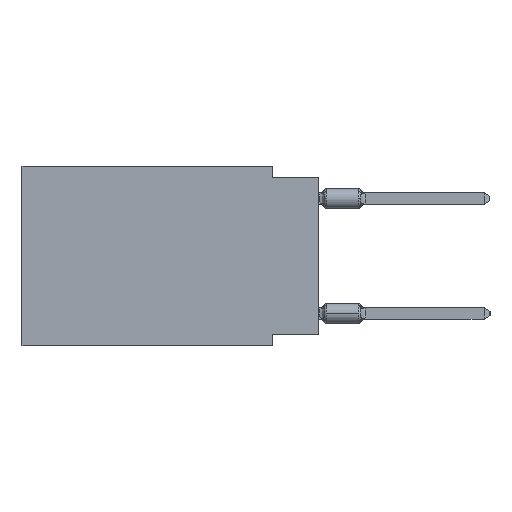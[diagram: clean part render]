
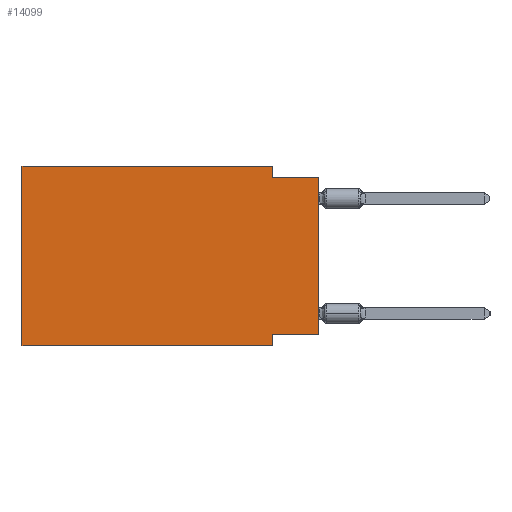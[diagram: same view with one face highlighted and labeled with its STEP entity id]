
A CAD part, left-side view. The second image highlights one B-rep face of the part: STEP entity #14099.
In plain terms, the highlighted planar face has unit normal (-1, 0, 0).
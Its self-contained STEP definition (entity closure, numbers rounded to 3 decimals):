
#2084 = ORIENTED_EDGE ( 'NONE', *, *, #8883, .F. ) ;
#2265 = VERTEX_POINT ( 'NONE', #6997 ) ;
#2411 = LINE ( 'NONE', #27732, #25319 ) ;
#3256 = DIRECTION ( 'NONE',  ( 0., -1., 0. ) ) ;
#3258 = ORIENTED_EDGE ( 'NONE', *, *, #47638, .T. ) ;
#3828 = VECTOR ( 'NONE', #37073, 1000. ) ;
#6430 = CARTESIAN_POINT ( 'NONE',  ( 0., 0., 0. ) ) ;
#6997 = CARTESIAN_POINT ( 'NONE',  ( 0., 2.54, -9.271 ) ) ;
#7080 = LINE ( 'NONE', #24614, #47276 ) ;
#8883 = EDGE_CURVE ( 'NONE', #46232, #43087, #38682, .T. ) ;
#8958 = EDGE_LOOP ( 'NONE', ( #43177, #30662, #22800, #29225, #2084, #3258, #28585, #29374 ) ) ;
#9475 = EDGE_CURVE ( 'NONE', #43087, #46721, #20190, .T. ) ;
#9549 = VECTOR ( 'NONE', #43375, 1000. ) ;
#9982 = LINE ( 'NONE', #18326, #9549 ) ;
#10958 = CARTESIAN_POINT ( 'NONE',  ( 0., 0., -9.271 ) ) ;
#11141 = EDGE_CURVE ( 'NONE', #47930, #27994, #48956, .T. ) ;
#13246 = VECTOR ( 'NONE', #52316, 1000. ) ;
#14099 = ADVANCED_FACE ( 'NONE', ( #23675 ), #27549, .F. ) ;
#14908 = CARTESIAN_POINT ( 'NONE',  ( 0., 16.383, 0. ) ) ;
#15680 = CARTESIAN_POINT ( 'NONE',  ( 0., 0., -9.271 ) ) ;
#15889 = CARTESIAN_POINT ( 'NONE',  ( 0., 16.383, 0. ) ) ;
#18326 = CARTESIAN_POINT ( 'NONE',  ( 0., 2.54, 0. ) ) ;
#19190 = EDGE_CURVE ( 'NONE', #36299, #27994, #53177, .T. ) ;
#19793 = DIRECTION ( 'NONE',  ( 0., 0., 1. ) ) ;
#20190 = LINE ( 'NONE', #14908, #28305 ) ;
#21902 = CARTESIAN_POINT ( 'NONE',  ( 0., 16.383, 0. ) ) ;
#22800 = ORIENTED_EDGE ( 'NONE', *, *, #40813, .F. ) ;
#22892 = CARTESIAN_POINT ( 'NONE',  ( 0., 2.54, 0. ) ) ;
#23675 = FACE_OUTER_BOUND ( 'NONE', #8958, .T. ) ;
#24413 = EDGE_CURVE ( 'NONE', #2265, #37347, #7080, .T. ) ;
#24614 = CARTESIAN_POINT ( 'NONE',  ( 0., 2.54, -9.906 ) ) ;
#25319 = VECTOR ( 'NONE', #3256, 1000. ) ;
#26107 = VECTOR ( 'NONE', #19793, 1000. ) ;
#27384 = VECTOR ( 'NONE', #39228, 1000. ) ;
#27549 = PLANE ( 'NONE',  #54284 ) ;
#27732 = CARTESIAN_POINT ( 'NONE',  ( 0., 16.383, -9.906 ) ) ;
#27994 = VERTEX_POINT ( 'NONE', #35067 ) ;
#28305 = VECTOR ( 'NONE', #37406, 1000. ) ;
#28585 = ORIENTED_EDGE ( 'NONE', *, *, #24413, .F. ) ;
#29225 = ORIENTED_EDGE ( 'NONE', *, *, #9475, .F. ) ;
#29374 = ORIENTED_EDGE ( 'NONE', *, *, #43826, .F. ) ;
#30662 = ORIENTED_EDGE ( 'NONE', *, *, #11141, .F. ) ;
#32063 = LINE ( 'NONE', #15680, #3828 ) ;
#35067 = CARTESIAN_POINT ( 'NONE',  ( 0., 0., -0.635 ) ) ;
#36299 = VERTEX_POINT ( 'NONE', #10958 ) ;
#36543 = DIRECTION ( 'NONE',  ( 0., 0., -1. ) ) ;
#37073 = DIRECTION ( 'NONE',  ( 0., 1., 0. ) ) ;
#37347 = VERTEX_POINT ( 'NONE', #43529 ) ;
#37406 = DIRECTION ( 'NONE',  ( 0., -1., 0. ) ) ;
#38682 = LINE ( 'NONE', #47314, #27384 ) ;
#39228 = DIRECTION ( 'NONE',  ( 0., 0., 1. ) ) ;
#40067 = DIRECTION ( 'NONE',  ( 1., 0., 0. ) ) ;
#40813 = EDGE_CURVE ( 'NONE', #46721, #47930, #9982, .T. ) ;
#43087 = VERTEX_POINT ( 'NONE', #21902 ) ;
#43177 = ORIENTED_EDGE ( 'NONE', *, *, #19190, .T. ) ;
#43375 = DIRECTION ( 'NONE',  ( 0., 0., -1. ) ) ;
#43529 = CARTESIAN_POINT ( 'NONE',  ( 0., 2.54, -9.906 ) ) ;
#43676 = CARTESIAN_POINT ( 'NONE',  ( 0., 0., -0.635 ) ) ;
#43826 = EDGE_CURVE ( 'NONE', #36299, #2265, #32063, .T. ) ;
#44530 = DIRECTION ( 'NONE',  ( 0., 0., -1. ) ) ;
#46232 = VERTEX_POINT ( 'NONE', #48595 ) ;
#46721 = VERTEX_POINT ( 'NONE', #22892 ) ;
#47276 = VECTOR ( 'NONE', #36543, 1000. ) ;
#47314 = CARTESIAN_POINT ( 'NONE',  ( 0., 16.383, 0. ) ) ;
#47638 = EDGE_CURVE ( 'NONE', #46232, #37347, #2411, .T. ) ;
#47930 = VERTEX_POINT ( 'NONE', #53477 ) ;
#48595 = CARTESIAN_POINT ( 'NONE',  ( 0., 16.383, -9.906 ) ) ;
#48956 = LINE ( 'NONE', #43676, #13246 ) ;
#52316 = DIRECTION ( 'NONE',  ( 0., -1., 0. ) ) ;
#53177 = LINE ( 'NONE', #6430, #26107 ) ;
#53477 = CARTESIAN_POINT ( 'NONE',  ( 0., 2.54, -0.635 ) ) ;
#54284 = AXIS2_PLACEMENT_3D ( 'NONE', #15889, #40067, #44530 ) ;
